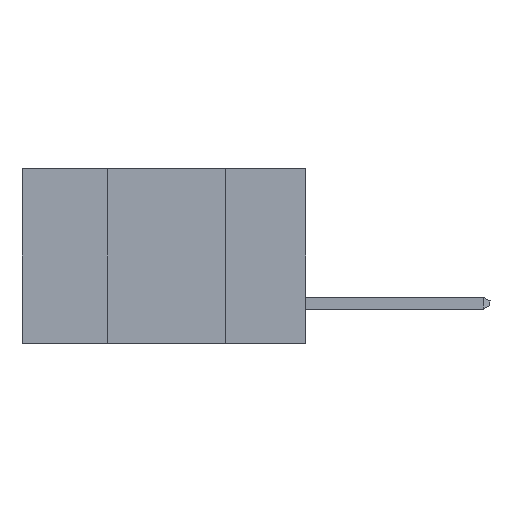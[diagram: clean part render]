
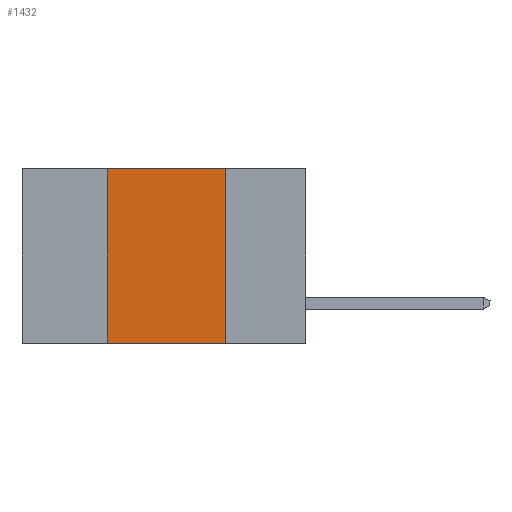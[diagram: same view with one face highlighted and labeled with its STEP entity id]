
A CAD part, left-side view. The second image highlights one B-rep face of the part: STEP entity #1432.
In plain terms, the highlighted planar face has unit normal (-1, 0, 0).
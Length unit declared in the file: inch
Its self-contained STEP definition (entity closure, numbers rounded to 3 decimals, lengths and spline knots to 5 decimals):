
#541 = VERTEX_POINT ( 'NONE', #9787 ) ;
#567 = CARTESIAN_POINT ( 'NONE',  ( 0., 0.6, -0.37 ) ) ;
#1432 = ADVANCED_FACE ( 'NONE', ( #4580 ), #3296, .F. ) ;
#1884 = EDGE_LOOP ( 'NONE', ( #9288, #6038, #1907, #5754 ) ) ;
#1907 = ORIENTED_EDGE ( 'NONE', *, *, #8142, .F. ) ;
#2314 = EDGE_CURVE ( 'NONE', #9534, #5940, #6655, .T. ) ;
#2768 = DIRECTION ( 'NONE',  ( 0., -1., 0. ) ) ;
#3296 = PLANE ( 'NONE',  #7990 ) ;
#4365 = CARTESIAN_POINT ( 'NONE',  ( 0., 0.42, 0. ) ) ;
#4580 = FACE_OUTER_BOUND ( 'NONE', #1884, .T. ) ;
#5056 = VECTOR ( 'NONE', #6339, 39.37008 ) ;
#5723 = CARTESIAN_POINT ( 'NONE',  ( 0., 0.42, -0.37 ) ) ;
#5754 = ORIENTED_EDGE ( 'NONE', *, *, #5807, .T. ) ;
#5766 = DIRECTION ( 'NONE',  ( 0., 0., -1. ) ) ;
#5807 = EDGE_CURVE ( 'NONE', #8301, #5940, #7789, .T. ) ;
#5888 = EDGE_CURVE ( 'NONE', #541, #9534, #12503, .T. ) ;
#5940 = VERTEX_POINT ( 'NONE', #12932 ) ;
#6038 = ORIENTED_EDGE ( 'NONE', *, *, #5888, .F. ) ;
#6339 = DIRECTION ( 'NONE',  ( 0., 0., 1. ) ) ;
#6354 = DIRECTION ( 'NONE',  ( 1., 0., 0. ) ) ;
#6655 = LINE ( 'NONE', #9966, #8856 ) ;
#7789 = LINE ( 'NONE', #567, #12838 ) ;
#7981 = CARTESIAN_POINT ( 'NONE',  ( 0., 0.6, 0. ) ) ;
#7990 = AXIS2_PLACEMENT_3D ( 'NONE', #12437, #6354, #11302 ) ;
#8142 = EDGE_CURVE ( 'NONE', #8301, #541, #8230, .T. ) ;
#8230 = LINE ( 'NONE', #4365, #5056 ) ;
#8301 = VERTEX_POINT ( 'NONE', #5723 ) ;
#8856 = VECTOR ( 'NONE', #5766, 39.37008 ) ;
#8966 = CARTESIAN_POINT ( 'NONE',  ( 0., 0.17, 0. ) ) ;
#9288 = ORIENTED_EDGE ( 'NONE', *, *, #2314, .F. ) ;
#9534 = VERTEX_POINT ( 'NONE', #8966 ) ;
#9787 = CARTESIAN_POINT ( 'NONE',  ( 0., 0.42, 0. ) ) ;
#9966 = CARTESIAN_POINT ( 'NONE',  ( 0., 0.17, 0. ) ) ;
#11057 = DIRECTION ( 'NONE',  ( 0., -1., 0. ) ) ;
#11302 = DIRECTION ( 'NONE',  ( 0., 0., -1. ) ) ;
#12197 = VECTOR ( 'NONE', #11057, 39.37008 ) ;
#12437 = CARTESIAN_POINT ( 'NONE',  ( 0., 0.6, 0. ) ) ;
#12503 = LINE ( 'NONE', #7981, #12197 ) ;
#12838 = VECTOR ( 'NONE', #2768, 39.37008 ) ;
#12932 = CARTESIAN_POINT ( 'NONE',  ( 0., 0.17, -0.37 ) ) ;
